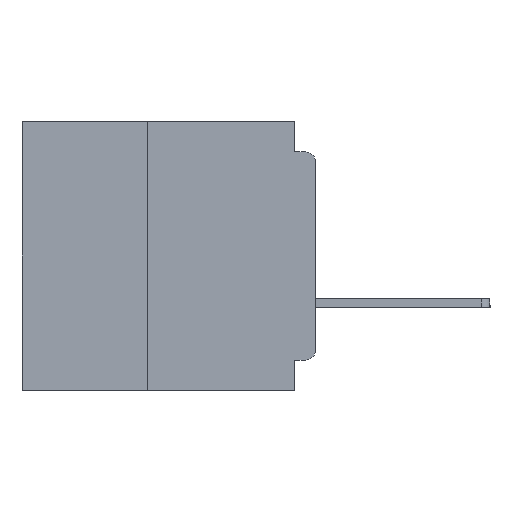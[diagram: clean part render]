
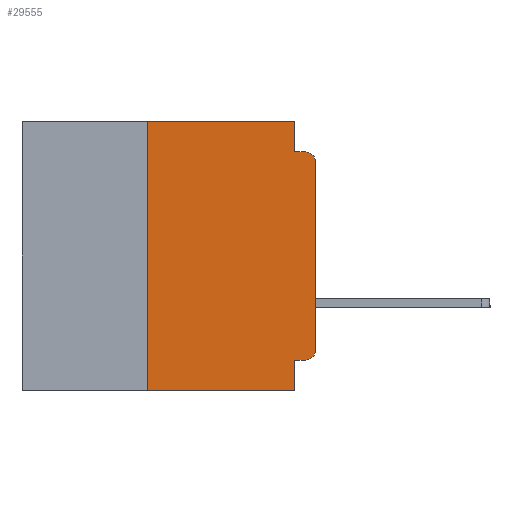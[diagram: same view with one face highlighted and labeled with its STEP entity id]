
A CAD part, left-side view. The second image highlights one B-rep face of the part: STEP entity #29555.
In plain terms, the highlighted planar face has unit normal (-1, 0, 0).
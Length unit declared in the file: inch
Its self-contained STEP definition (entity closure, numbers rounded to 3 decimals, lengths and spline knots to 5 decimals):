
#375 = ORIENTED_EDGE ( 'NONE', *, *, #6473, .T. ) ;
#1748 = VERTEX_POINT ( 'NONE', #2982 ) ;
#2982 = CARTESIAN_POINT ( 'NONE',  ( 0., 0.031, -0.045 ) ) ;
#3542 = VECTOR ( 'NONE', #3893, 39.37008 ) ;
#3548 = CARTESIAN_POINT ( 'NONE',  ( 0., 0.25, -0.4 ) ) ;
#3609 = DIRECTION ( 'NONE',  ( 0., 0., -1. ) ) ;
#3893 = DIRECTION ( 'NONE',  ( 0., -1., 0. ) ) ;
#4361 = DIRECTION ( 'NONE',  ( 0., 0., -1. ) ) ;
#4869 = CIRCLE ( 'NONE', #35915, 0.015 ) ;
#5541 = DIRECTION ( 'NONE',  ( 0., 0., 1. ) ) ;
#5598 = VERTEX_POINT ( 'NONE', #30518 ) ;
#5775 = AXIS2_PLACEMENT_3D ( 'NONE', #39432, #15475, #43364 ) ;
#6473 = EDGE_CURVE ( 'NONE', #48879, #17237, #4869, .T. ) ;
#8354 = ORIENTED_EDGE ( 'NONE', *, *, #49962, .F. ) ;
#8703 = VERTEX_POINT ( 'NONE', #23429 ) ;
#10172 = EDGE_CURVE ( 'NONE', #37639, #48879, #13187, .T. ) ;
#10630 = EDGE_CURVE ( 'NONE', #50682, #1748, #35722, .T. ) ;
#11010 = CARTESIAN_POINT ( 'NONE',  ( 0., 0.437, -0.4 ) ) ;
#12082 = VECTOR ( 'NONE', #15082, 39.37008 ) ;
#12720 = CARTESIAN_POINT ( 'NONE',  ( 0., 0.031, 0. ) ) ;
#12888 = ORIENTED_EDGE ( 'NONE', *, *, #45617, .F. ) ;
#13187 = LINE ( 'NONE', #25831, #33293 ) ;
#14342 = EDGE_CURVE ( 'NONE', #39649, #18028, #21580, .T. ) ;
#15082 = DIRECTION ( 'NONE',  ( 0., -1., 0. ) ) ;
#15133 = CARTESIAN_POINT ( 'NONE',  ( 0., 0.437, 0. ) ) ;
#15475 = DIRECTION ( 'NONE',  ( -1., 0., 0. ) ) ;
#15596 = CARTESIAN_POINT ( 'NONE',  ( 0., 0.437, 0. ) ) ;
#16313 = EDGE_CURVE ( 'NONE', #34959, #50682, #17596, .T. ) ;
#16368 = ORIENTED_EDGE ( 'NONE', *, *, #10172, .T. ) ;
#16655 = CARTESIAN_POINT ( 'NONE',  ( 0., 0., -0.34 ) ) ;
#17237 = VERTEX_POINT ( 'NONE', #49609 ) ;
#17596 = LINE ( 'NONE', #15133, #27060 ) ;
#18028 = VERTEX_POINT ( 'NONE', #38747 ) ;
#19780 = EDGE_CURVE ( 'NONE', #39649, #34959, #42144, .T. ) ;
#20343 = CARTESIAN_POINT ( 'NONE',  ( 0., 0.031, 0. ) ) ;
#20649 = CARTESIAN_POINT ( 'NONE',  ( 0., 0.015, -0.06 ) ) ;
#20993 = VECTOR ( 'NONE', #24307, 39.37008 ) ;
#21580 = LINE ( 'NONE', #11010, #12082 ) ;
#23429 = CARTESIAN_POINT ( 'NONE',  ( 0., 0.031, -0.355 ) ) ;
#23918 = VECTOR ( 'NONE', #44119, 39.37008 ) ;
#24307 = DIRECTION ( 'NONE',  ( 0., 0., 1. ) ) ;
#24694 = DIRECTION ( 'NONE',  ( 0., 0., -1. ) ) ;
#24856 = ORIENTED_EDGE ( 'NONE', *, *, #19780, .F. ) ;
#25006 = LINE ( 'NONE', #32050, #3542 ) ;
#25422 = EDGE_CURVE ( 'NONE', #5598, #8703, #43271, .T. ) ;
#25831 = CARTESIAN_POINT ( 'NONE',  ( 0., 0., 0. ) ) ;
#25941 = VECTOR ( 'NONE', #30855, 39.37008 ) ;
#26234 = ORIENTED_EDGE ( 'NONE', *, *, #10630, .F. ) ;
#26721 = FACE_OUTER_BOUND ( 'NONE', #29364, .T. ) ;
#26868 = CARTESIAN_POINT ( 'NONE',  ( 0., 0., -0.355 ) ) ;
#27060 = VECTOR ( 'NONE', #50903, 39.37008 ) ;
#27777 = DIRECTION ( 'NONE',  ( 1., 0., 0. ) ) ;
#29364 = EDGE_LOOP ( 'NONE', ( #16368, #375, #12888, #26234, #48943, #24856, #51393, #8354, #37027, #32636 ) ) ;
#29555 = ADVANCED_FACE ( 'NONE', ( #26721 ), #51345, .F. ) ;
#30518 = CARTESIAN_POINT ( 'NONE',  ( 0., 0.015, -0.355 ) ) ;
#30855 = DIRECTION ( 'NONE',  ( 0., 1., 0. ) ) ;
#32050 = CARTESIAN_POINT ( 'NONE',  ( 0., 0., -0.045 ) ) ;
#32636 = ORIENTED_EDGE ( 'NONE', *, *, #47563, .T. ) ;
#32984 = AXIS2_PLACEMENT_3D ( 'NONE', #15596, #27777, #3609 ) ;
#33293 = VECTOR ( 'NONE', #5541, 39.37008 ) ;
#34959 = VERTEX_POINT ( 'NONE', #50545 ) ;
#35722 = LINE ( 'NONE', #20343, #23918 ) ;
#35915 = AXIS2_PLACEMENT_3D ( 'NONE', #20649, #48335, #24694 ) ;
#36438 = CARTESIAN_POINT ( 'NONE',  ( 0., 0.031, -0.4 ) ) ;
#36672 = CARTESIAN_POINT ( 'NONE',  ( 0., 0., -0.06 ) ) ;
#37027 = ORIENTED_EDGE ( 'NONE', *, *, #25422, .F. ) ;
#37639 = VERTEX_POINT ( 'NONE', #16655 ) ;
#38747 = CARTESIAN_POINT ( 'NONE',  ( 0., 0.031, -0.4 ) ) ;
#39432 = CARTESIAN_POINT ( 'NONE',  ( 0., 0.015, -0.34 ) ) ;
#39649 = VERTEX_POINT ( 'NONE', #3548 ) ;
#39908 = LINE ( 'NONE', #36438, #50306 ) ;
#42144 = LINE ( 'NONE', #47956, #20993 ) ;
#43271 = LINE ( 'NONE', #26868, #25941 ) ;
#43364 = DIRECTION ( 'NONE',  ( 0., 0., -1. ) ) ;
#44119 = DIRECTION ( 'NONE',  ( 0., 0., -1. ) ) ;
#45617 = EDGE_CURVE ( 'NONE', #1748, #17237, #25006, .T. ) ;
#47563 = EDGE_CURVE ( 'NONE', #5598, #37639, #47583, .T. ) ;
#47583 = CIRCLE ( 'NONE', #5775, 0.015 ) ;
#47956 = CARTESIAN_POINT ( 'NONE',  ( 0., 0.25, -0.4 ) ) ;
#48335 = DIRECTION ( 'NONE',  ( -1., 0., 0. ) ) ;
#48879 = VERTEX_POINT ( 'NONE', #36672 ) ;
#48943 = ORIENTED_EDGE ( 'NONE', *, *, #16313, .F. ) ;
#49609 = CARTESIAN_POINT ( 'NONE',  ( 0., 0.015, -0.045 ) ) ;
#49962 = EDGE_CURVE ( 'NONE', #8703, #18028, #39908, .T. ) ;
#50306 = VECTOR ( 'NONE', #4361, 39.37008 ) ;
#50545 = CARTESIAN_POINT ( 'NONE',  ( 0., 0.25, 0. ) ) ;
#50682 = VERTEX_POINT ( 'NONE', #12720 ) ;
#50903 = DIRECTION ( 'NONE',  ( 0., -1., 0. ) ) ;
#51345 = PLANE ( 'NONE',  #32984 ) ;
#51393 = ORIENTED_EDGE ( 'NONE', *, *, #14342, .T. ) ;
